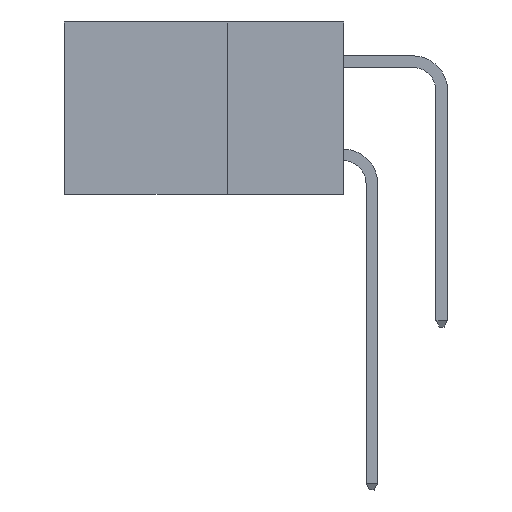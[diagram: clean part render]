
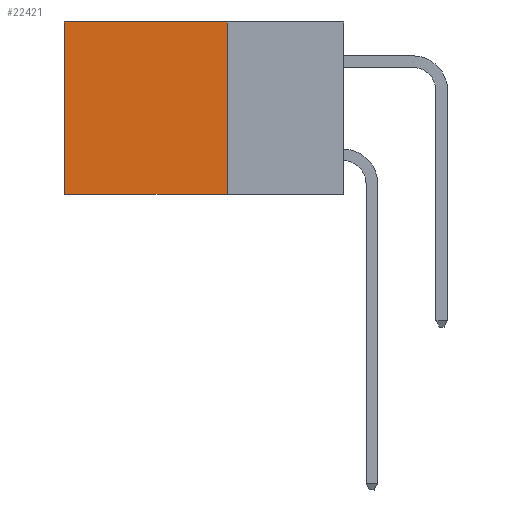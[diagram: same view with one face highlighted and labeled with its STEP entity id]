
A CAD part, left-side view. The second image highlights one B-rep face of the part: STEP entity #22421.
In plain terms, the highlighted planar face has unit normal (-1, 0, 0).
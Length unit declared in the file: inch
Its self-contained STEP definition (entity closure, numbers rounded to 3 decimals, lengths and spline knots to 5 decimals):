
#110 = CARTESIAN_POINT ( 'NONE',  ( 0.2615, 0.25, -0.37 ) ) ;
#410 = LINE ( 'NONE', #18743, #3842 ) ;
#1406 = CARTESIAN_POINT ( 'NONE',  ( 0.2615, 0.25, -0.37 ) ) ;
#1741 = VERTEX_POINT ( 'NONE', #19299 ) ;
#2147 = DIRECTION ( 'NONE',  ( 0., 0., -1. ) ) ;
#2379 = ORIENTED_EDGE ( 'NONE', *, *, #24682, .F. ) ;
#2487 = EDGE_CURVE ( 'NONE', #13996, #12080, #14431, .T. ) ;
#3842 = VECTOR ( 'NONE', #2147, 39.37008 ) ;
#4637 = VERTEX_POINT ( 'NONE', #20396 ) ;
#6809 = AXIS2_PLACEMENT_3D ( 'NONE', #1406, #26176, #17859 ) ;
#6966 = ORIENTED_EDGE ( 'NONE', *, *, #26220, .T. ) ;
#8281 = LINE ( 'NONE', #18488, #10210 ) ;
#9104 = LINE ( 'NONE', #15404, #16837 ) ;
#9695 = PLANE ( 'NONE',  #6809 ) ;
#10210 = VECTOR ( 'NONE', #20489, 39.37008 ) ;
#11204 = VECTOR ( 'NONE', #22594, 39.37008 ) ;
#11708 = FACE_OUTER_BOUND ( 'NONE', #13896, .T. ) ;
#12080 = VERTEX_POINT ( 'NONE', #21374 ) ;
#13896 = EDGE_LOOP ( 'NONE', ( #6966, #19516, #2379, #24795 ) ) ;
#13996 = VERTEX_POINT ( 'NONE', #22523 ) ;
#14431 = LINE ( 'NONE', #110, #11204 ) ;
#15118 = DIRECTION ( 'NONE',  ( 0., 0., -1. ) ) ;
#15138 = EDGE_CURVE ( 'NONE', #1741, #4637, #8281, .T. ) ;
#15404 = CARTESIAN_POINT ( 'NONE',  ( 0.2615, 0.6, -0.37 ) ) ;
#16837 = VECTOR ( 'NONE', #15118, 39.37008 ) ;
#17859 = DIRECTION ( 'NONE',  ( 0., 0., -1. ) ) ;
#18488 = CARTESIAN_POINT ( 'NONE',  ( 0.2615, 0.25, 0. ) ) ;
#18743 = CARTESIAN_POINT ( 'NONE',  ( 0.2615, 0.25, -0.37 ) ) ;
#19299 = CARTESIAN_POINT ( 'NONE',  ( 0.2615, 0.25, 0. ) ) ;
#19516 = ORIENTED_EDGE ( 'NONE', *, *, #2487, .F. ) ;
#20396 = CARTESIAN_POINT ( 'NONE',  ( 0.2615, 0.6, 0. ) ) ;
#20489 = DIRECTION ( 'NONE',  ( 0., 1., 0. ) ) ;
#21374 = CARTESIAN_POINT ( 'NONE',  ( 0.2615, 0.6, -0.37 ) ) ;
#22421 = ADVANCED_FACE ( 'NONE', ( #11708 ), #9695, .F. ) ;
#22523 = CARTESIAN_POINT ( 'NONE',  ( 0.2615, 0.25, -0.37 ) ) ;
#22594 = DIRECTION ( 'NONE',  ( 0., 1., 0. ) ) ;
#24682 = EDGE_CURVE ( 'NONE', #1741, #13996, #410, .T. ) ;
#24795 = ORIENTED_EDGE ( 'NONE', *, *, #15138, .T. ) ;
#26176 = DIRECTION ( 'NONE',  ( 1., 0., 0. ) ) ;
#26220 = EDGE_CURVE ( 'NONE', #4637, #12080, #9104, .T. ) ;
